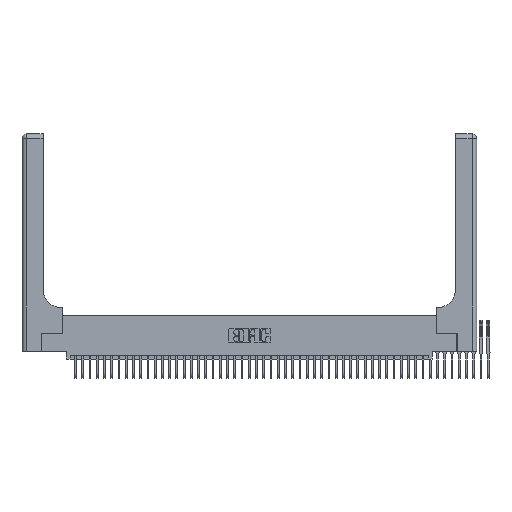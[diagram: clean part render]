
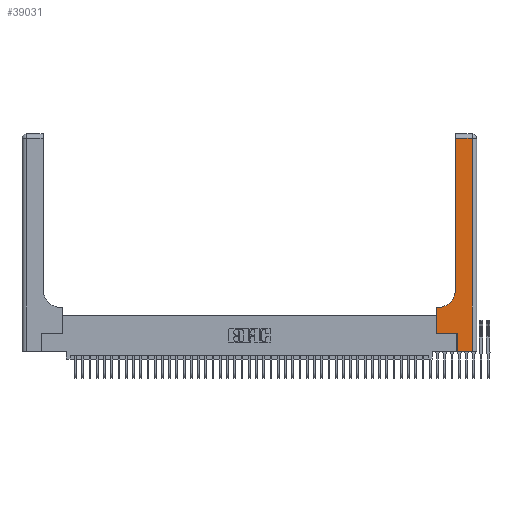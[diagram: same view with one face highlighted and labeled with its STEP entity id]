
A CAD part, top view. The second image highlights one B-rep face of the part: STEP entity #39031.
In plain terms, the highlighted face is planar.
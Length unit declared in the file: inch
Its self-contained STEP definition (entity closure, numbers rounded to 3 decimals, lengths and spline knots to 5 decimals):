
#567 = CARTESIAN_POINT ( 'NONE',  ( 0., 0., 0. ) ) ;
#1113 = ORIENTED_EDGE ( 'NONE', *, *, #34252, .F. ) ;
#1374 = VECTOR ( 'NONE', #24395, 39.37008 ) ;
#1701 = CARTESIAN_POINT ( 'NONE',  ( 0.2915, 2.94, 0. ) ) ;
#2173 = CARTESIAN_POINT ( 'NONE',  ( 0.269, 0.25, 0. ) ) ;
#2604 = CARTESIAN_POINT ( 'NONE',  ( 0.5585, 0.25, 0. ) ) ;
#3383 = PLANE ( 'NONE',  #17587 ) ;
#4540 = ORIENTED_EDGE ( 'NONE', *, *, #5553, .F. ) ;
#5075 = ORIENTED_EDGE ( 'NONE', *, *, #16386, .F. ) ;
#5553 = EDGE_CURVE ( 'NONE', #21873, #26955, #11996, .T. ) ;
#5576 = EDGE_CURVE ( 'NONE', #13679, #22047, #10002, .T. ) ;
#5676 = VECTOR ( 'NONE', #10357, 39.37008 ) ;
#7006 = CARTESIAN_POINT ( 'NONE',  ( 0.269, 0., 0. ) ) ;
#7218 = VERTEX_POINT ( 'NONE', #7006 ) ;
#7948 = CARTESIAN_POINT ( 'NONE',  ( 0.06, 0., 0. ) ) ;
#9889 = CARTESIAN_POINT ( 'NONE',  ( 0., 3., 0. ) ) ;
#10002 = LINE ( 'NONE', #17932, #1374 ) ;
#10357 = DIRECTION ( 'NONE',  ( 1., 0., 0. ) ) ;
#10864 = EDGE_LOOP ( 'NONE', ( #37446, #36712, #38202, #31339, #4540, #1113, #19598, #5075, #26402 ) ) ;
#10973 = CARTESIAN_POINT ( 'NONE',  ( 0.5415, 0.6, 0. ) ) ;
#11440 = VECTOR ( 'NONE', #39543, 39.37008 ) ;
#11600 = VERTEX_POINT ( 'NONE', #21657 ) ;
#11996 = LINE ( 'NONE', #21032, #12998 ) ;
#12695 = EDGE_CURVE ( 'NONE', #11600, #13003, #28747, .T. ) ;
#12998 = VECTOR ( 'NONE', #33856, 39.37008 ) ;
#13003 = VERTEX_POINT ( 'NONE', #13573 ) ;
#13050 = VECTOR ( 'NONE', #21870, 39.37008 ) ;
#13094 = DIRECTION ( 'NONE',  ( -1., 0., 0. ) ) ;
#13153 = CIRCLE ( 'NONE', #21108, 0.25 ) ;
#13573 = CARTESIAN_POINT ( 'NONE',  ( 0.5585, 0.25, 0. ) ) ;
#13679 = VERTEX_POINT ( 'NONE', #21979 ) ;
#13817 = VECTOR ( 'NONE', #23972, 39.37008 ) ;
#14250 = LINE ( 'NONE', #567, #5676 ) ;
#14923 = VECTOR ( 'NONE', #41442, 39.37008 ) ;
#15457 = CARTESIAN_POINT ( 'NONE',  ( 0.5415, 0.85, 0. ) ) ;
#15557 = EDGE_CURVE ( 'NONE', #40661, #13679, #40484, .T. ) ;
#16386 = EDGE_CURVE ( 'NONE', #7218, #11600, #22340, .T. ) ;
#17587 = AXIS2_PLACEMENT_3D ( 'NONE', #9889, #32407, #13094 ) ;
#17932 = CARTESIAN_POINT ( 'NONE',  ( 0.2915, 2.94, 0. ) ) ;
#18684 = DIRECTION ( 'NONE',  ( 1., 0., 0. ) ) ;
#19598 = ORIENTED_EDGE ( 'NONE', *, *, #12695, .F. ) ;
#20032 = CARTESIAN_POINT ( 'NONE',  ( 0.5585, 0.6, 0. ) ) ;
#20189 = VECTOR ( 'NONE', #37746, 39.37008 ) ;
#20401 = EDGE_CURVE ( 'NONE', #32429, #22047, #28539, .T. ) ;
#21032 = CARTESIAN_POINT ( 'NONE',  ( 0.2915, 0.6, 0. ) ) ;
#21108 = AXIS2_PLACEMENT_3D ( 'NONE', #15457, #37935, #18684 ) ;
#21657 = CARTESIAN_POINT ( 'NONE',  ( 0.269, 0.25, 0. ) ) ;
#21870 = DIRECTION ( 'NONE',  ( 0., 1., 0. ) ) ;
#21873 = VERTEX_POINT ( 'NONE', #20032 ) ;
#21979 = CARTESIAN_POINT ( 'NONE',  ( 0.06, 2.94, 0. ) ) ;
#22047 = VERTEX_POINT ( 'NONE', #1701 ) ;
#22340 = LINE ( 'NONE', #33578, #13817 ) ;
#23425 = CARTESIAN_POINT ( 'NONE',  ( 0.2915, 3., 0. ) ) ;
#23972 = DIRECTION ( 'NONE',  ( 0., 1., 0. ) ) ;
#24395 = DIRECTION ( 'NONE',  ( 1., 0., 0. ) ) ;
#26402 = ORIENTED_EDGE ( 'NONE', *, *, #38486, .F. ) ;
#26955 = VERTEX_POINT ( 'NONE', #10973 ) ;
#28274 = FACE_OUTER_BOUND ( 'NONE', #10864, .T. ) ;
#28539 = LINE ( 'NONE', #23425, #11440 ) ;
#28747 = LINE ( 'NONE', #2173, #20189 ) ;
#31101 = CARTESIAN_POINT ( 'NONE',  ( 0.2915, 0.85, 0. ) ) ;
#31191 = LINE ( 'NONE', #2604, #13050 ) ;
#31339 = ORIENTED_EDGE ( 'NONE', *, *, #39475, .F. ) ;
#32407 = DIRECTION ( 'NONE',  ( 0., 0., -1. ) ) ;
#32429 = VERTEX_POINT ( 'NONE', #31101 ) ;
#33578 = CARTESIAN_POINT ( 'NONE',  ( 0.269, 0., 0. ) ) ;
#33856 = DIRECTION ( 'NONE',  ( -1., 0., 0. ) ) ;
#34252 = EDGE_CURVE ( 'NONE', #13003, #21873, #31191, .T. ) ;
#35064 = CARTESIAN_POINT ( 'NONE',  ( 0.06, 3., 0. ) ) ;
#36712 = ORIENTED_EDGE ( 'NONE', *, *, #5576, .T. ) ;
#37446 = ORIENTED_EDGE ( 'NONE', *, *, #15557, .T. ) ;
#37746 = DIRECTION ( 'NONE',  ( 1., 0., 0. ) ) ;
#37935 = DIRECTION ( 'NONE',  ( 0., 0., -1. ) ) ;
#38202 = ORIENTED_EDGE ( 'NONE', *, *, #20401, .F. ) ;
#38486 = EDGE_CURVE ( 'NONE', #40661, #7218, #14250, .T. ) ;
#39031 = ADVANCED_FACE ( 'NONE', ( #28274 ), #3383, .T. ) ;
#39475 = EDGE_CURVE ( 'NONE', #26955, #32429, #13153, .T. ) ;
#39543 = DIRECTION ( 'NONE',  ( 0., 1., 0. ) ) ;
#40484 = LINE ( 'NONE', #35064, #14923 ) ;
#40661 = VERTEX_POINT ( 'NONE', #7948 ) ;
#41442 = DIRECTION ( 'NONE',  ( 0., 1., 0. ) ) ;
